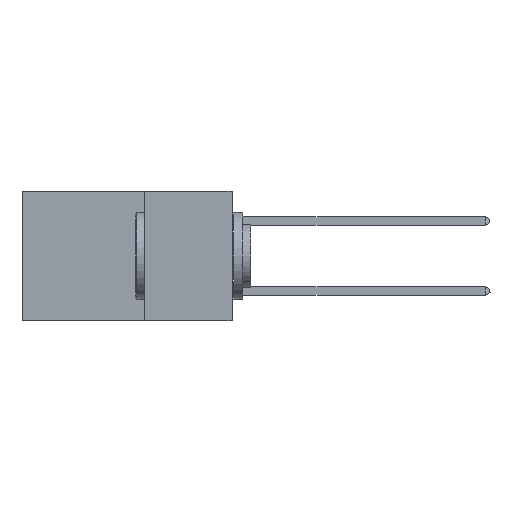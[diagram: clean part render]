
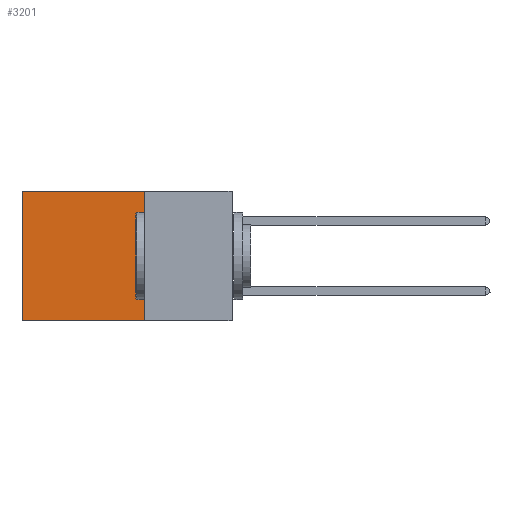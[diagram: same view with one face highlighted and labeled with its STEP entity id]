
A CAD part, left-side view. The second image highlights one B-rep face of the part: STEP entity #3201.
In plain terms, the highlighted planar face has unit normal (-1, 0, 0).
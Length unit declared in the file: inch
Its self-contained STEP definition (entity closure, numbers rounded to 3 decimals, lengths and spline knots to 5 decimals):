
#611 = VERTEX_POINT ( 'NONE', #4265 ) ;
#1407 = EDGE_CURVE ( 'NONE', #6716, #2676, #10611, .T. ) ;
#1410 = VECTOR ( 'NONE', #6988, 39.37008 ) ;
#1534 = VECTOR ( 'NONE', #14078, 39.37008 ) ;
#1919 = DIRECTION ( 'NONE',  ( 0., 0., -1. ) ) ;
#2365 = VERTEX_POINT ( 'NONE', #10459 ) ;
#2377 = DIRECTION ( 'NONE',  ( 0., 0., -1. ) ) ;
#2419 = DIRECTION ( 'NONE',  ( 1., 0., 0. ) ) ;
#2487 = CARTESIAN_POINT ( 'NONE',  ( 0.2875, 0.25, 0. ) ) ;
#2495 = PLANE ( 'NONE',  #12958 ) ;
#2510 = VECTOR ( 'NONE', #1919, 39.37008 ) ;
#2676 = VERTEX_POINT ( 'NONE', #7269 ) ;
#3138 = CARTESIAN_POINT ( 'NONE',  ( 0.2875, 0.25, 0. ) ) ;
#3201 = ADVANCED_FACE ( 'NONE', ( #6429 ), #2495, .F. ) ;
#3444 = DIRECTION ( 'NONE',  ( 0., 1., 0. ) ) ;
#4265 = CARTESIAN_POINT ( 'NONE',  ( 0.2875, 0.25, -0.37 ) ) ;
#4457 = CARTESIAN_POINT ( 'NONE',  ( 0.2875, 0.25, 0. ) ) ;
#5142 = ORIENTED_EDGE ( 'NONE', *, *, #1407, .T. ) ;
#5499 = EDGE_CURVE ( 'NONE', #611, #2365, #14306, .T. ) ;
#6056 = ORIENTED_EDGE ( 'NONE', *, *, #5499, .F. ) ;
#6429 = FACE_OUTER_BOUND ( 'NONE', #7549, .T. ) ;
#6716 = VERTEX_POINT ( 'NONE', #6751 ) ;
#6751 = CARTESIAN_POINT ( 'NONE',  ( 0.2875, 0.25, 0. ) ) ;
#6988 = DIRECTION ( 'NONE',  ( 0., 0., -1. ) ) ;
#7269 = CARTESIAN_POINT ( 'NONE',  ( 0.2875, 0.6, 0. ) ) ;
#7549 = EDGE_LOOP ( 'NONE', ( #13862, #6056, #10264, #5142 ) ) ;
#7619 = VECTOR ( 'NONE', #3444, 39.37008 ) ;
#10264 = ORIENTED_EDGE ( 'NONE', *, *, #10618, .F. ) ;
#10459 = CARTESIAN_POINT ( 'NONE',  ( 0.2875, 0.6, -0.37 ) ) ;
#10611 = LINE ( 'NONE', #3138, #7619 ) ;
#10618 = EDGE_CURVE ( 'NONE', #6716, #611, #14773, .T. ) ;
#10870 = LINE ( 'NONE', #11535, #1410 ) ;
#11535 = CARTESIAN_POINT ( 'NONE',  ( 0.2875, 0.6, 0. ) ) ;
#12958 = AXIS2_PLACEMENT_3D ( 'NONE', #2487, #2419, #2377 ) ;
#13862 = ORIENTED_EDGE ( 'NONE', *, *, #14189, .T. ) ;
#14078 = DIRECTION ( 'NONE',  ( 0., 1., 0. ) ) ;
#14189 = EDGE_CURVE ( 'NONE', #2676, #2365, #10870, .T. ) ;
#14207 = CARTESIAN_POINT ( 'NONE',  ( 0.2875, 0.25, -0.37 ) ) ;
#14306 = LINE ( 'NONE', #14207, #1534 ) ;
#14773 = LINE ( 'NONE', #4457, #2510 ) ;
